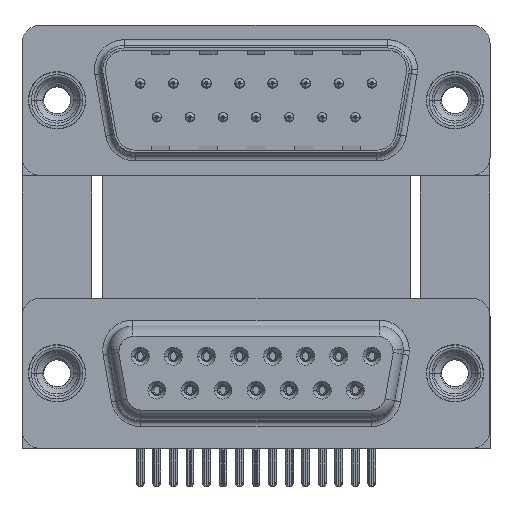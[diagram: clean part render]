
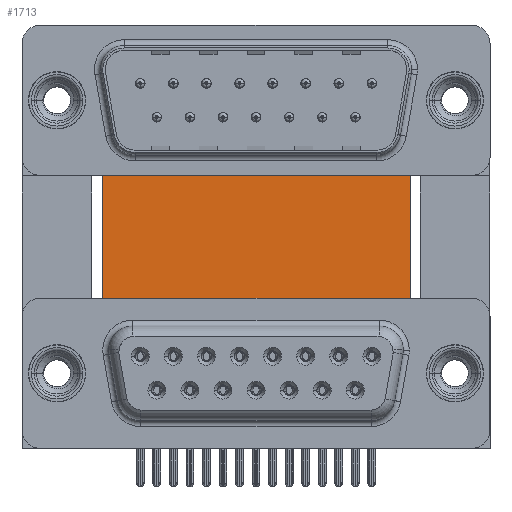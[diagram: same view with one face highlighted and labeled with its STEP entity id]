
A CAD part, top view. The second image highlights one B-rep face of the part: STEP entity #1713.
In plain terms, the highlighted planar face has unit normal (0, 0, 1).
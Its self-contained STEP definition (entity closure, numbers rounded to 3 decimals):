
#1713 = ADVANCED_FACE ( 'NONE', ( #21210 ), #14329, .F. ) ;
#2246 = DIRECTION ( 'NONE',  ( 1., 0., 0. ) ) ;
#4554 = DIRECTION ( 'NONE',  ( 0., -1., 0. ) ) ;
#4607 = EDGE_CURVE ( 'NONE', #34874, #7434, #7103, .T. ) ;
#4685 = VECTOR ( 'NONE', #41316, 1000. ) ;
#4930 = CARTESIAN_POINT ( 'NONE',  ( 29.58, -3.735, -12. ) ) ;
#6824 = DIRECTION ( 'NONE',  ( 1., 0., 0. ) ) ;
#7103 = LINE ( 'NONE', #28997, #4685 ) ;
#7434 = VERTEX_POINT ( 'NONE', #4930 ) ;
#9137 = ORIENTED_EDGE ( 'NONE', *, *, #24643, .T. ) ;
#13529 = CARTESIAN_POINT ( 'NONE',  ( 3.79, -3.735, -12. ) ) ;
#13900 = DIRECTION ( 'NONE',  ( 0., 0., -1. ) ) ;
#14329 = PLANE ( 'NONE',  #30776 ) ;
#15540 = EDGE_CURVE ( 'NONE', #27853, #34874, #16130, .T. ) ;
#16130 = LINE ( 'NONE', #40612, #27464 ) ;
#17843 = VERTEX_POINT ( 'NONE', #13529 ) ;
#18217 = EDGE_CURVE ( 'NONE', #17843, #7434, #21810, .T. ) ;
#18691 = CARTESIAN_POINT ( 'NONE',  ( 3.79, -3.735, -12. ) ) ;
#19548 = ORIENTED_EDGE ( 'NONE', *, *, #18217, .T. ) ;
#20359 = ORIENTED_EDGE ( 'NONE', *, *, #15540, .F. ) ;
#21210 = FACE_OUTER_BOUND ( 'NONE', #40979, .T. ) ;
#21440 = ORIENTED_EDGE ( 'NONE', *, *, #4607, .F. ) ;
#21810 = LINE ( 'NONE', #18691, #34053 ) ;
#24643 = EDGE_CURVE ( 'NONE', #27853, #17843, #32091, .T. ) ;
#24991 = DIRECTION ( 'NONE',  ( -1., 0., 0. ) ) ;
#27464 = VECTOR ( 'NONE', #6824, 1000. ) ;
#27853 = VERTEX_POINT ( 'NONE', #42427 ) ;
#28997 = CARTESIAN_POINT ( 'NONE',  ( 29.58, 16.585, -12. ) ) ;
#30776 = AXIS2_PLACEMENT_3D ( 'NONE', #35007, #13900, #24991 ) ;
#31652 = CARTESIAN_POINT ( 'NONE',  ( 3.79, 16.585, -12. ) ) ;
#32091 = LINE ( 'NONE', #31652, #35718 ) ;
#34053 = VECTOR ( 'NONE', #2246, 1000. ) ;
#34874 = VERTEX_POINT ( 'NONE', #36107 ) ;
#35007 = CARTESIAN_POINT ( 'NONE',  ( 3.79, 16.585, -12. ) ) ;
#35718 = VECTOR ( 'NONE', #4554, 1000. ) ;
#36107 = CARTESIAN_POINT ( 'NONE',  ( 29.58, 16.585, -12. ) ) ;
#40612 = CARTESIAN_POINT ( 'NONE',  ( 3.79, 16.585, -12. ) ) ;
#40979 = EDGE_LOOP ( 'NONE', ( #19548, #21440, #20359, #9137 ) ) ;
#41316 = DIRECTION ( 'NONE',  ( 0., -1., 0. ) ) ;
#42427 = CARTESIAN_POINT ( 'NONE',  ( 3.79, 16.585, -12. ) ) ;
